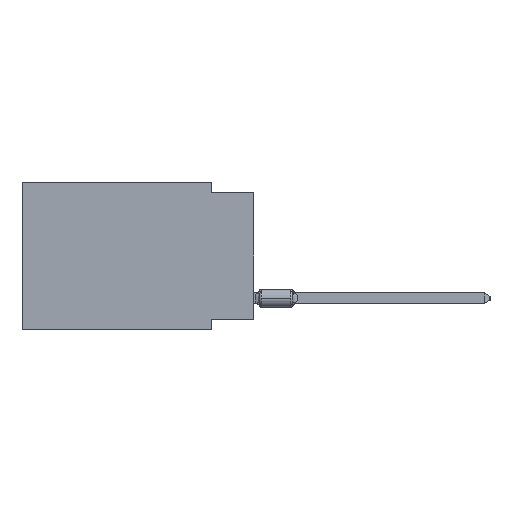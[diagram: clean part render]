
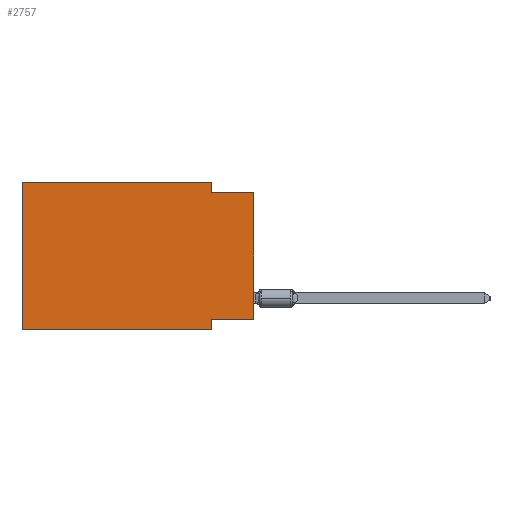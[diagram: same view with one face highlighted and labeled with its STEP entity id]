
A CAD part, left-side view. The second image highlights one B-rep face of the part: STEP entity #2757.
In plain terms, the highlighted planar face has unit normal (-1, 0, 0).
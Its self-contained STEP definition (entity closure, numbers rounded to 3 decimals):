
#1063 = CARTESIAN_POINT ( 'NONE',  ( 0., 13.97, 0. ) ) ;
#1295 = CARTESIAN_POINT ( 'NONE',  ( 0., 0., 0. ) ) ;
#1411 = LINE ( 'NONE', #19948, #16463 ) ;
#1495 = ORIENTED_EDGE ( 'NONE', *, *, #32594, .F. ) ;
#1636 = CARTESIAN_POINT ( 'NONE',  ( 0., 13.97, 0. ) ) ;
#1863 = ORIENTED_EDGE ( 'NONE', *, *, #28192, .T. ) ;
#2166 = VECTOR ( 'NONE', #6328, 1000. ) ;
#2174 = DIRECTION ( 'NONE',  ( 0., 0., 1. ) ) ;
#2757 = ADVANCED_FACE ( 'NONE', ( #17620 ), #25993, .F. ) ;
#3163 = EDGE_CURVE ( 'NONE', #6335, #14121, #23030, .T. ) ;
#4111 = CARTESIAN_POINT ( 'NONE',  ( 0., 2.54, -8.89 ) ) ;
#5437 = CARTESIAN_POINT ( 'NONE',  ( 0., 0., -8.255 ) ) ;
#5447 = CARTESIAN_POINT ( 'NONE',  ( 0., 0., -0.635 ) ) ;
#6065 = VECTOR ( 'NONE', #20646, 1000. ) ;
#6226 = ORIENTED_EDGE ( 'NONE', *, *, #9860, .F. ) ;
#6328 = DIRECTION ( 'NONE',  ( 0., 1., 0. ) ) ;
#6335 = VERTEX_POINT ( 'NONE', #7890 ) ;
#6509 = LINE ( 'NONE', #11610, #2166 ) ;
#6694 = DIRECTION ( 'NONE',  ( 1., 0., 0. ) ) ;
#6839 = DIRECTION ( 'NONE',  ( 0., -1., 0. ) ) ;
#7364 = ORIENTED_EDGE ( 'NONE', *, *, #34099, .F. ) ;
#7890 = CARTESIAN_POINT ( 'NONE',  ( 0., 2.54, -0.635 ) ) ;
#7916 = CARTESIAN_POINT ( 'NONE',  ( 0., 13.97, -8.89 ) ) ;
#7955 = CARTESIAN_POINT ( 'NONE',  ( 0., 2.54, -8.255 ) ) ;
#8641 = LINE ( 'NONE', #28307, #20255 ) ;
#9797 = EDGE_CURVE ( 'NONE', #20168, #35852, #8641, .T. ) ;
#9860 = EDGE_CURVE ( 'NONE', #23911, #33013, #25571, .T. ) ;
#10307 = CARTESIAN_POINT ( 'NONE',  ( 0., 2.54, 0. ) ) ;
#11077 = DIRECTION ( 'NONE',  ( 0., 0., 1. ) ) ;
#11610 = CARTESIAN_POINT ( 'NONE',  ( 0., 0., -8.255 ) ) ;
#13790 = EDGE_LOOP ( 'NONE', ( #1863, #28029, #7364, #6226, #1495, #32271, #32150, #16670 ) ) ;
#14121 = VERTEX_POINT ( 'NONE', #5447 ) ;
#15583 = VERTEX_POINT ( 'NONE', #7955 ) ;
#16463 = VECTOR ( 'NONE', #31812, 1000. ) ;
#16670 = ORIENTED_EDGE ( 'NONE', *, *, #28409, .F. ) ;
#17620 = FACE_OUTER_BOUND ( 'NONE', #13790, .T. ) ;
#17718 = AXIS2_PLACEMENT_3D ( 'NONE', #1063, #6694, #20525 ) ;
#17811 = VECTOR ( 'NONE', #6839, 1000. ) ;
#19948 = CARTESIAN_POINT ( 'NONE',  ( 0., 2.54, 0. ) ) ;
#20168 = VERTEX_POINT ( 'NONE', #7916 ) ;
#20255 = VECTOR ( 'NONE', #24673, 1000. ) ;
#20525 = DIRECTION ( 'NONE',  ( 0., 0., -1. ) ) ;
#20646 = DIRECTION ( 'NONE',  ( 0., -1., 0. ) ) ;
#20709 = VECTOR ( 'NONE', #11077, 1000. ) ;
#23030 = LINE ( 'NONE', #34148, #17811 ) ;
#23850 = LINE ( 'NONE', #34777, #25983 ) ;
#23911 = VERTEX_POINT ( 'NONE', #29899 ) ;
#24673 = DIRECTION ( 'NONE',  ( 0., -1., 0. ) ) ;
#25571 = LINE ( 'NONE', #34682, #6065 ) ;
#25983 = VECTOR ( 'NONE', #26771, 1000. ) ;
#25993 = PLANE ( 'NONE',  #17718 ) ;
#26231 = LINE ( 'NONE', #1295, #20709 ) ;
#26771 = DIRECTION ( 'NONE',  ( 0., 0., -1. ) ) ;
#27108 = LINE ( 'NONE', #1636, #35438 ) ;
#28029 = ORIENTED_EDGE ( 'NONE', *, *, #3163, .F. ) ;
#28192 = EDGE_CURVE ( 'NONE', #31763, #14121, #26231, .T. ) ;
#28307 = CARTESIAN_POINT ( 'NONE',  ( 0., 13.97, -8.89 ) ) ;
#28409 = EDGE_CURVE ( 'NONE', #31763, #15583, #6509, .T. ) ;
#29899 = CARTESIAN_POINT ( 'NONE',  ( 0., 13.97, 0. ) ) ;
#30424 = EDGE_CURVE ( 'NONE', #15583, #35852, #23850, .T. ) ;
#31763 = VERTEX_POINT ( 'NONE', #5437 ) ;
#31812 = DIRECTION ( 'NONE',  ( 0., 0., -1. ) ) ;
#32150 = ORIENTED_EDGE ( 'NONE', *, *, #30424, .F. ) ;
#32271 = ORIENTED_EDGE ( 'NONE', *, *, #9797, .T. ) ;
#32594 = EDGE_CURVE ( 'NONE', #20168, #23911, #27108, .T. ) ;
#33013 = VERTEX_POINT ( 'NONE', #10307 ) ;
#34099 = EDGE_CURVE ( 'NONE', #33013, #6335, #1411, .T. ) ;
#34148 = CARTESIAN_POINT ( 'NONE',  ( 0., 0., -0.635 ) ) ;
#34682 = CARTESIAN_POINT ( 'NONE',  ( 0., 13.97, 0. ) ) ;
#34777 = CARTESIAN_POINT ( 'NONE',  ( 0., 2.54, -8.89 ) ) ;
#35438 = VECTOR ( 'NONE', #2174, 1000. ) ;
#35852 = VERTEX_POINT ( 'NONE', #4111 ) ;
